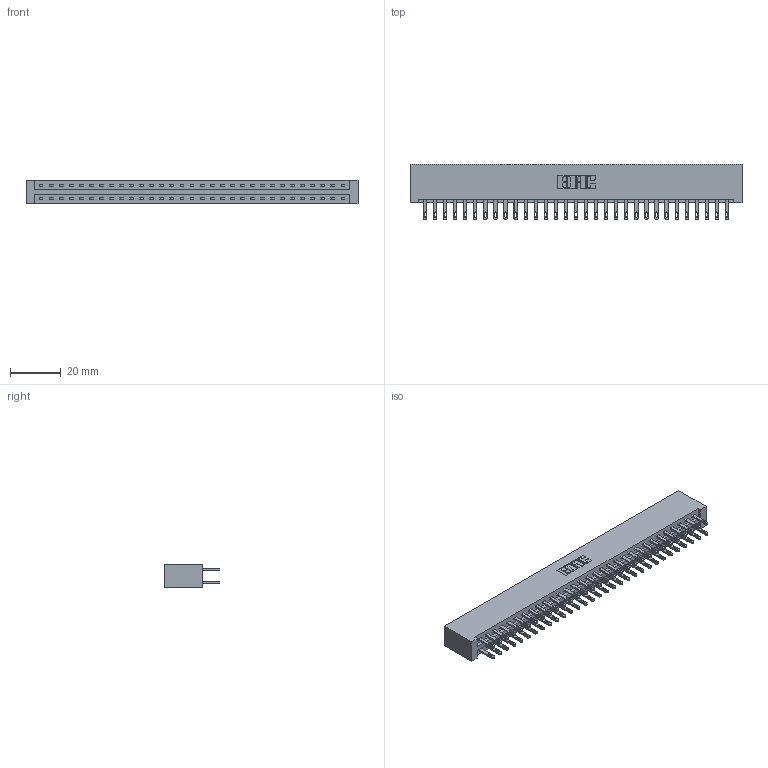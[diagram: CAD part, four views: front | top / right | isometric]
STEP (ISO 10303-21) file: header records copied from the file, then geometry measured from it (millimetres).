
FILE_DESCRIPTION (( 'STEP AP203' ), '1' );
FILE_NAME ('337-062-500-201.STEP', '2018-08-10T09:28:38', ( '' ), ( '' ), 'SwSTEP 2.0', 'SolidWorks 2016', '' );
FILE_SCHEMA (( 'CONFIG_CONTROL_DESIGN' ));
Length unit declared in the file: inch
Products named in the file (3): 345-292-001_345-293-100; 337-062-500-201; 337 Part_No Mounting Lugs
Assembly tree (63 placements, depth 2):
  337-062-500-201
    337 Part_No Mounting Lugs
    345-292-001_345-293-100  x62
Bounding box: 130.71 x 21.85 x 9.4 mm (x, y, z)
Volume: 14578.9 mm3; surface area: 17118.6 mm2
Topology: 63 solids, 63 shells, 3206 faces, 9773 edges, 6514 vertices
Faces by surface type: plane 2050, cylinder 1156
Entity records: 25111 total; most frequent: CARTESIAN_POINT 4238, ORIENTED_EDGE 4174, DIRECTION 3619, EDGE_CURVE 2087, LINE 1963, VECTOR 1963, VERTEX_POINT 1390, AXIS2_PLACEMENT_3D 828
